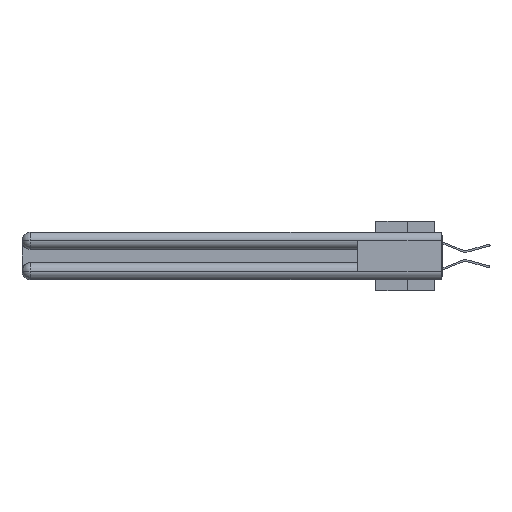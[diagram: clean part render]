
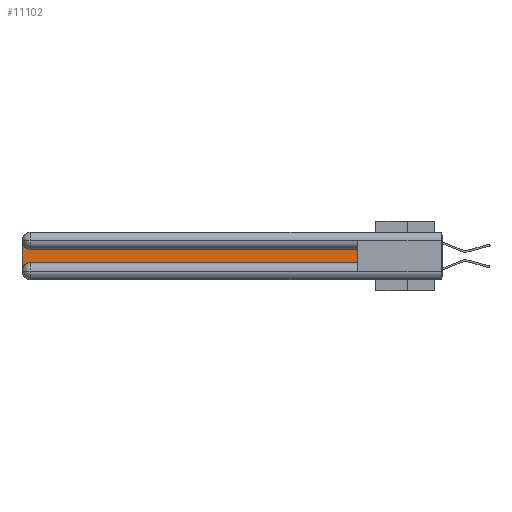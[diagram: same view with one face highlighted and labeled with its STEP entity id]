
A CAD part, left-side view. The second image highlights one B-rep face of the part: STEP entity #11102.
In plain terms, the highlighted planar face has unit normal (-1, 0, 0).
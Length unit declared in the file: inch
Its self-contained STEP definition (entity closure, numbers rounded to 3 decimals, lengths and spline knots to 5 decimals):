
#26 = CARTESIAN_POINT ( 'NONE',  ( 0.075, 2.94, -0.2175 ) ) ;
#63 = EDGE_CURVE ( 'NONE', #24546, #13233, #5601, .T. ) ;
#1592 = DIRECTION ( 'NONE',  ( 1., 0., 0. ) ) ;
#2957 = DIRECTION ( 'NONE',  ( 1., 0., 0. ) ) ;
#4212 = CIRCLE ( 'NONE', #26481, 0.06 ) ;
#4319 = CARTESIAN_POINT ( 'NONE',  ( 0.075, 3., -0.1225 ) ) ;
#5366 = CIRCLE ( 'NONE', #11622, 0.06 ) ;
#5555 = DIRECTION ( 'NONE',  ( 0., 1., 0. ) ) ;
#5601 = LINE ( 'NONE', #17553, #11059 ) ;
#6061 = CARTESIAN_POINT ( 'NONE',  ( 0.075, 0.6, -0.1225 ) ) ;
#6272 = VECTOR ( 'NONE', #29901, 39.37008 ) ;
#6718 = AXIS2_PLACEMENT_3D ( 'NONE', #4319, #20640, #13681 ) ;
#7342 = LINE ( 'NONE', #29813, #6272 ) ;
#7434 = VERTEX_POINT ( 'NONE', #23006 ) ;
#7465 = DIRECTION ( 'NONE',  ( 0., 0., -1. ) ) ;
#8670 = ORIENTED_EDGE ( 'NONE', *, *, #29333, .T. ) ;
#9007 = EDGE_CURVE ( 'NONE', #13233, #21238, #15935, .T. ) ;
#9029 = VERTEX_POINT ( 'NONE', #15188 ) ;
#9823 = CARTESIAN_POINT ( 'NONE',  ( 0.075, 3., -0.2775 ) ) ;
#11059 = VECTOR ( 'NONE', #24700, 39.37008 ) ;
#11102 = ADVANCED_FACE ( 'NONE', ( #22220 ), #13459, .F. ) ;
#11622 = AXIS2_PLACEMENT_3D ( 'NONE', #20559, #1592, #13398 ) ;
#12507 = LINE ( 'NONE', #17372, #26020 ) ;
#13233 = VERTEX_POINT ( 'NONE', #18129 ) ;
#13398 = DIRECTION ( 'NONE',  ( 0., 0., -1. ) ) ;
#13459 = PLANE ( 'NONE',  #6718 ) ;
#13681 = DIRECTION ( 'NONE',  ( 0., 0., -1. ) ) ;
#13739 = VECTOR ( 'NONE', #24291, 39.37008 ) ;
#14712 = ORIENTED_EDGE ( 'NONE', *, *, #15265, .T. ) ;
#15188 = CARTESIAN_POINT ( 'NONE',  ( 0.075, 2.94, -0.1225 ) ) ;
#15265 = EDGE_CURVE ( 'NONE', #21238, #9029, #12507, .T. ) ;
#15935 = LINE ( 'NONE', #17767, #13739 ) ;
#16650 = EDGE_LOOP ( 'NONE', ( #14712, #28323, #26788, #8670, #24127, #20641 ) ) ;
#17265 = VERTEX_POINT ( 'NONE', #9823 ) ;
#17372 = CARTESIAN_POINT ( 'NONE',  ( 0.075, 0.6, -0.1225 ) ) ;
#17553 = CARTESIAN_POINT ( 'NONE',  ( 0.075, 0.6, -0.2175 ) ) ;
#17767 = CARTESIAN_POINT ( 'NONE',  ( 0.075, 0.6, -0.2175 ) ) ;
#18129 = CARTESIAN_POINT ( 'NONE',  ( 0.075, 0.6, -0.2175 ) ) ;
#20559 = CARTESIAN_POINT ( 'NONE',  ( 0.075, 2.94, -0.2775 ) ) ;
#20640 = DIRECTION ( 'NONE',  ( 1., 0., 0. ) ) ;
#20641 = ORIENTED_EDGE ( 'NONE', *, *, #9007, .T. ) ;
#21238 = VERTEX_POINT ( 'NONE', #6061 ) ;
#21529 = CARTESIAN_POINT ( 'NONE',  ( 0.075, 2.94, -0.0625 ) ) ;
#22220 = FACE_OUTER_BOUND ( 'NONE', #16650, .T. ) ;
#23006 = CARTESIAN_POINT ( 'NONE',  ( 0.075, 3., -0.0625 ) ) ;
#24127 = ORIENTED_EDGE ( 'NONE', *, *, #63, .T. ) ;
#24291 = DIRECTION ( 'NONE',  ( 0., 0., 1. ) ) ;
#24546 = VERTEX_POINT ( 'NONE', #26 ) ;
#24700 = DIRECTION ( 'NONE',  ( 0., -1., 0. ) ) ;
#25049 = EDGE_CURVE ( 'NONE', #7434, #17265, #7342, .T. ) ;
#26020 = VECTOR ( 'NONE', #5555, 39.37008 ) ;
#26481 = AXIS2_PLACEMENT_3D ( 'NONE', #21529, #2957, #7465 ) ;
#26788 = ORIENTED_EDGE ( 'NONE', *, *, #25049, .T. ) ;
#28323 = ORIENTED_EDGE ( 'NONE', *, *, #30148, .T. ) ;
#29333 = EDGE_CURVE ( 'NONE', #17265, #24546, #5366, .T. ) ;
#29813 = CARTESIAN_POINT ( 'NONE',  ( 0.075, 3., -0.2175 ) ) ;
#29901 = DIRECTION ( 'NONE',  ( 0., 0., -1. ) ) ;
#30148 = EDGE_CURVE ( 'NONE', #9029, #7434, #4212, .T. ) ;
